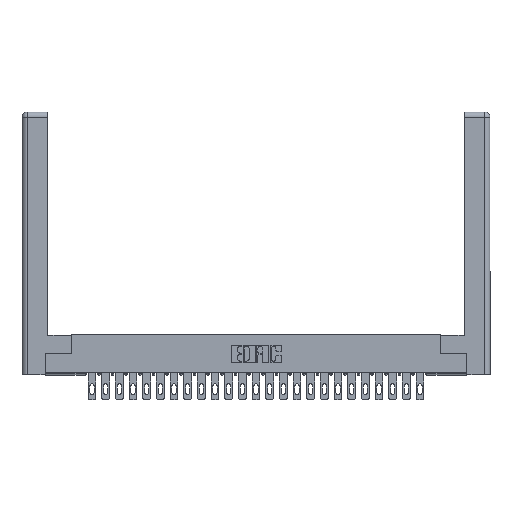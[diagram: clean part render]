
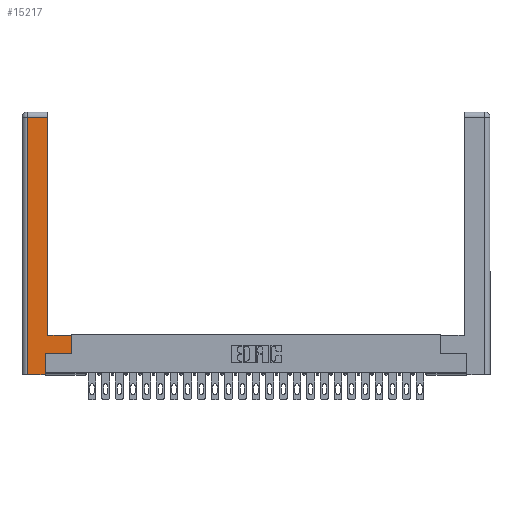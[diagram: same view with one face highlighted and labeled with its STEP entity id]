
A CAD part, top view. The second image highlights one B-rep face of the part: STEP entity #15217.
In plain terms, the highlighted planar face has unit normal (0, 0, 1).
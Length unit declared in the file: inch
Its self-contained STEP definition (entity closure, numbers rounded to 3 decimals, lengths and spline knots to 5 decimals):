
#90 = EDGE_CURVE ( 'NONE', #13333, #13517, #3342, .T. ) ;
#1245 = EDGE_CURVE ( 'NONE', #18731, #21234, #8654, .T. ) ;
#1384 = LINE ( 'NONE', #26779, #15265 ) ;
#1670 = CARTESIAN_POINT ( 'NONE',  ( 0.565, 0.45, 0. ) ) ;
#2841 = ORIENTED_EDGE ( 'NONE', *, *, #1245, .T. ) ;
#3024 = VECTOR ( 'NONE', #16013, 39.37008 ) ;
#3027 = VERTEX_POINT ( 'NONE', #7454 ) ;
#3342 = LINE ( 'NONE', #27736, #13014 ) ;
#3827 = VERTEX_POINT ( 'NONE', #11741 ) ;
#4590 = VECTOR ( 'NONE', #27245, 39.37008 ) ;
#4944 = VERTEX_POINT ( 'NONE', #14601 ) ;
#4959 = CARTESIAN_POINT ( 'NONE',  ( 0.0615, 2.94, 0. ) ) ;
#5078 = DIRECTION ( 'NONE',  ( -1., 0., 0. ) ) ;
#5459 = EDGE_CURVE ( 'NONE', #4944, #18731, #18115, .T. ) ;
#6601 = DIRECTION ( 'NONE',  ( 0., 1., 0. ) ) ;
#7262 = DIRECTION ( 'NONE',  ( -1., 0., 0. ) ) ;
#7390 = EDGE_CURVE ( 'NONE', #21234, #3027, #1384, .T. ) ;
#7454 = CARTESIAN_POINT ( 'NONE',  ( 0.295, 0.45, 0. ) ) ;
#8078 = LINE ( 'NONE', #29505, #20449 ) ;
#8654 = LINE ( 'NONE', #1670, #29433 ) ;
#8831 = EDGE_CURVE ( 'NONE', #3827, #9171, #25554, .T. ) ;
#9171 = VERTEX_POINT ( 'NONE', #21461 ) ;
#9640 = PLANE ( 'NONE',  #11176 ) ;
#10730 = EDGE_LOOP ( 'NONE', ( #18198, #29842, #23762, #11703, #24757, #26252, #2841, #20329 ) ) ;
#11143 = LINE ( 'NONE', #29925, #4590 ) ;
#11176 = AXIS2_PLACEMENT_3D ( 'NONE', #13659, #17200, #7262 ) ;
#11703 = ORIENTED_EDGE ( 'NONE', *, *, #90, .T. ) ;
#11741 = CARTESIAN_POINT ( 'NONE',  ( 0.295, 2.94, 0. ) ) ;
#12780 = LINE ( 'NONE', #27843, #30809 ) ;
#12951 = DIRECTION ( 'NONE',  ( 0., 1., 0. ) ) ;
#13014 = VECTOR ( 'NONE', #15320, 39.37008 ) ;
#13332 = CARTESIAN_POINT ( 'NONE',  ( 0.265, 0., 0. ) ) ;
#13333 = VERTEX_POINT ( 'NONE', #24838 ) ;
#13517 = VERTEX_POINT ( 'NONE', #13332 ) ;
#13535 = CARTESIAN_POINT ( 'NONE',  ( 0.565, 0.245, 0. ) ) ;
#13659 = CARTESIAN_POINT ( 'NONE',  ( 0., 0., 0. ) ) ;
#13669 = VECTOR ( 'NONE', #5078, 39.37008 ) ;
#14601 = CARTESIAN_POINT ( 'NONE',  ( 0.265, 0.245, 0. ) ) ;
#14857 = FACE_OUTER_BOUND ( 'NONE', #10730, .T. ) ;
#15217 = ADVANCED_FACE ( 'NONE', ( #14857 ), #9640, .F. ) ;
#15265 = VECTOR ( 'NONE', #31708, 39.37008 ) ;
#15320 = DIRECTION ( 'NONE',  ( 1., 0., 0. ) ) ;
#15974 = EDGE_CURVE ( 'NONE', #9171, #13333, #8078, .T. ) ;
#16013 = DIRECTION ( 'NONE',  ( 1., 0., 0. ) ) ;
#16856 = CARTESIAN_POINT ( 'NONE',  ( 0.565, 0.245, 0. ) ) ;
#17200 = DIRECTION ( 'NONE',  ( 0., 0., -1. ) ) ;
#18115 = LINE ( 'NONE', #13535, #3024 ) ;
#18198 = ORIENTED_EDGE ( 'NONE', *, *, #21485, .T. ) ;
#18731 = VERTEX_POINT ( 'NONE', #16856 ) ;
#20329 = ORIENTED_EDGE ( 'NONE', *, *, #7390, .T. ) ;
#20449 = VECTOR ( 'NONE', #29387, 39.37008 ) ;
#21234 = VERTEX_POINT ( 'NONE', #23664 ) ;
#21461 = CARTESIAN_POINT ( 'NONE',  ( 0.0615, 2.94, 0. ) ) ;
#21485 = EDGE_CURVE ( 'NONE', #3027, #3827, #12780, .T. ) ;
#23664 = CARTESIAN_POINT ( 'NONE',  ( 0.565, 0.45, 0. ) ) ;
#23762 = ORIENTED_EDGE ( 'NONE', *, *, #15974, .T. ) ;
#24757 = ORIENTED_EDGE ( 'NONE', *, *, #29840, .T. ) ;
#24838 = CARTESIAN_POINT ( 'NONE',  ( 0.0615, 0., 0. ) ) ;
#25554 = LINE ( 'NONE', #4959, #13669 ) ;
#26252 = ORIENTED_EDGE ( 'NONE', *, *, #5459, .T. ) ;
#26779 = CARTESIAN_POINT ( 'NONE',  ( 0.295, 0.45, 0. ) ) ;
#27245 = DIRECTION ( 'NONE',  ( 0., 1., 0. ) ) ;
#27736 = CARTESIAN_POINT ( 'NONE',  ( 0.265, 0., 0. ) ) ;
#27843 = CARTESIAN_POINT ( 'NONE',  ( 0.295, 3., 0. ) ) ;
#29387 = DIRECTION ( 'NONE',  ( 0., -1., 0. ) ) ;
#29433 = VECTOR ( 'NONE', #6601, 39.37008 ) ;
#29505 = CARTESIAN_POINT ( 'NONE',  ( 0.0615, 0., 0. ) ) ;
#29840 = EDGE_CURVE ( 'NONE', #13517, #4944, #11143, .T. ) ;
#29842 = ORIENTED_EDGE ( 'NONE', *, *, #8831, .T. ) ;
#29925 = CARTESIAN_POINT ( 'NONE',  ( 0.265, 0.245, 0. ) ) ;
#30809 = VECTOR ( 'NONE', #12951, 39.37008 ) ;
#31708 = DIRECTION ( 'NONE',  ( -1., 0., 0. ) ) ;
